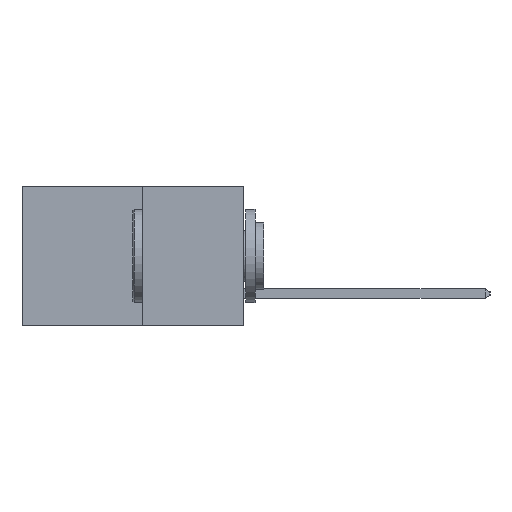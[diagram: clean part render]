
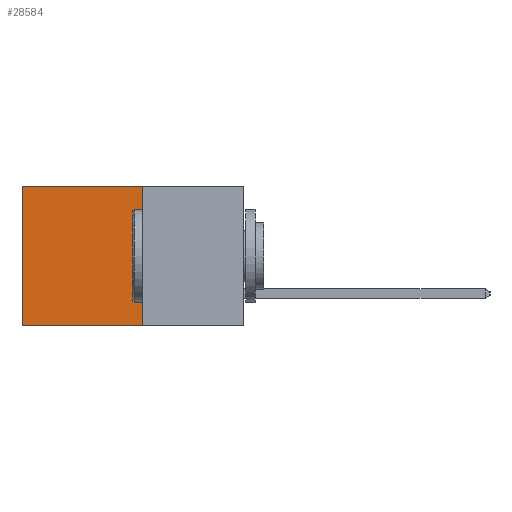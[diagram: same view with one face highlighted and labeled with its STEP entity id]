
A CAD part, left-side view. The second image highlights one B-rep face of the part: STEP entity #28584.
In plain terms, the highlighted planar face has unit normal (-1, 0, 0).
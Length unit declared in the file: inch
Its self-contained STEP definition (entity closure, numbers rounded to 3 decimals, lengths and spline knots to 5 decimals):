
#3104 = FACE_OUTER_BOUND ( 'NONE', #7255, .T. ) ;
#3716 = ORIENTED_EDGE ( 'NONE', *, *, #26646, .T. ) ;
#3916 = CARTESIAN_POINT ( 'NONE',  ( 0.277, 0.27, 0. ) ) ;
#3958 = AXIS2_PLACEMENT_3D ( 'NONE', #10107, #12540, #29161 ) ;
#7255 = EDGE_LOOP ( 'NONE', ( #14270, #9358, #22155, #3716 ) ) ;
#7653 = PLANE ( 'NONE',  #3958 ) ;
#7848 = VERTEX_POINT ( 'NONE', #23605 ) ;
#9358 = ORIENTED_EDGE ( 'NONE', *, *, #10028, .F. ) ;
#9607 = LINE ( 'NONE', #10212, #21646 ) ;
#10028 = EDGE_CURVE ( 'NONE', #16517, #25797, #18041, .T. ) ;
#10107 = CARTESIAN_POINT ( 'NONE',  ( 0.277, 0.27, -0.37 ) ) ;
#10212 = CARTESIAN_POINT ( 'NONE',  ( 0.277, 0.27, 0. ) ) ;
#11916 = CARTESIAN_POINT ( 'NONE',  ( 0.277, 0.27, -0.37 ) ) ;
#12540 = DIRECTION ( 'NONE',  ( 1., 0., 0. ) ) ;
#12588 = VECTOR ( 'NONE', #14311, 39.37008 ) ;
#14205 = VERTEX_POINT ( 'NONE', #3916 ) ;
#14270 = ORIENTED_EDGE ( 'NONE', *, *, #24248, .T. ) ;
#14311 = DIRECTION ( 'NONE',  ( 0., 0., -1. ) ) ;
#15358 = CARTESIAN_POINT ( 'NONE',  ( 0.277, 0.27, -0.37 ) ) ;
#16517 = VERTEX_POINT ( 'NONE', #15358 ) ;
#17490 = CARTESIAN_POINT ( 'NONE',  ( 0.277, 0.27, -0.37 ) ) ;
#18041 = LINE ( 'NONE', #17490, #23577 ) ;
#21646 = VECTOR ( 'NONE', #26909, 39.37008 ) ;
#22155 = ORIENTED_EDGE ( 'NONE', *, *, #28403, .F. ) ;
#23378 = CARTESIAN_POINT ( 'NONE',  ( 0.277, 0.59, -0.37 ) ) ;
#23577 = VECTOR ( 'NONE', #24627, 39.37008 ) ;
#23605 = CARTESIAN_POINT ( 'NONE',  ( 0.277, 0.59, 0. ) ) ;
#24248 = EDGE_CURVE ( 'NONE', #7848, #25797, #30622, .T. ) ;
#24627 = DIRECTION ( 'NONE',  ( 0., 1., 0. ) ) ;
#25167 = VECTOR ( 'NONE', #25759, 39.37008 ) ;
#25759 = DIRECTION ( 'NONE',  ( 0., 0., -1. ) ) ;
#25797 = VERTEX_POINT ( 'NONE', #26132 ) ;
#26006 = LINE ( 'NONE', #11916, #12588 ) ;
#26132 = CARTESIAN_POINT ( 'NONE',  ( 0.277, 0.59, -0.37 ) ) ;
#26646 = EDGE_CURVE ( 'NONE', #14205, #7848, #9607, .T. ) ;
#26909 = DIRECTION ( 'NONE',  ( 0., 1., 0. ) ) ;
#28403 = EDGE_CURVE ( 'NONE', #14205, #16517, #26006, .T. ) ;
#28584 = ADVANCED_FACE ( 'NONE', ( #3104 ), #7653, .F. ) ;
#29161 = DIRECTION ( 'NONE',  ( 0., 0., -1. ) ) ;
#30622 = LINE ( 'NONE', #23378, #25167 ) ;
